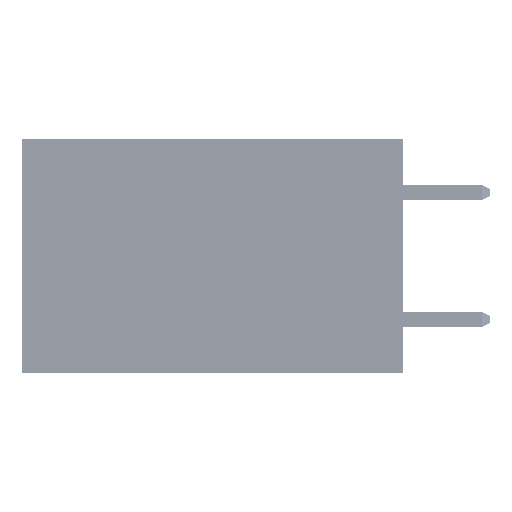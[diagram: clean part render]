
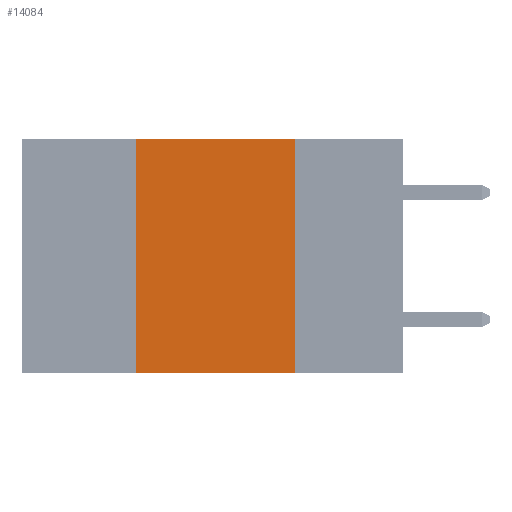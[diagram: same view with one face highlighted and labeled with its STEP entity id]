
A CAD part, left-side view. The second image highlights one B-rep face of the part: STEP entity #14084.
In plain terms, the highlighted planar face has unit normal (-1, 0, 0).
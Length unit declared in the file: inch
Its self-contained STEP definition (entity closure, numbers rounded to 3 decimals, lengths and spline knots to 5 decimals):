
#609 = CARTESIAN_POINT ( 'NONE',  ( 0., 0.17, 0. ) ) ;
#5768 = LINE ( 'NONE', #37172, #46860 ) ;
#5972 = ORIENTED_EDGE ( 'NONE', *, *, #36355, .F. ) ;
#6825 = ORIENTED_EDGE ( 'NONE', *, *, #26324, .F. ) ;
#8878 = CARTESIAN_POINT ( 'NONE',  ( 0., 0.17, 0. ) ) ;
#10198 = AXIS2_PLACEMENT_3D ( 'NONE', #22796, #34400, #19366 ) ;
#10320 = FACE_OUTER_BOUND ( 'NONE', #25816, .T. ) ;
#14084 = ADVANCED_FACE ( 'NONE', ( #10320 ), #42012, .F. ) ;
#14096 = VERTEX_POINT ( 'NONE', #609 ) ;
#15864 = CARTESIAN_POINT ( 'NONE',  ( 0., 0.42, 0. ) ) ;
#15959 = CARTESIAN_POINT ( 'NONE',  ( 0., 0.42, 0. ) ) ;
#18615 = VERTEX_POINT ( 'NONE', #35736 ) ;
#19366 = DIRECTION ( 'NONE',  ( 0., 0., -1. ) ) ;
#19368 = CARTESIAN_POINT ( 'NONE',  ( 0., 0.6, 0. ) ) ;
#19670 = VERTEX_POINT ( 'NONE', #29926 ) ;
#19706 = EDGE_CURVE ( 'NONE', #18615, #19670, #5768, .T. ) ;
#20727 = DIRECTION ( 'NONE',  ( 0., 0., -1. ) ) ;
#22165 = LINE ( 'NONE', #19368, #46283 ) ;
#22796 = CARTESIAN_POINT ( 'NONE',  ( 0., 0.6, 0. ) ) ;
#23823 = DIRECTION ( 'NONE',  ( 0., 0., 1. ) ) ;
#23917 = LINE ( 'NONE', #15864, #33580 ) ;
#25816 = EDGE_LOOP ( 'NONE', ( #42036, #5972, #6825, #30201 ) ) ;
#26324 = EDGE_CURVE ( 'NONE', #18615, #44539, #23917, .T. ) ;
#26517 = DIRECTION ( 'NONE',  ( 0., -1., 0. ) ) ;
#28520 = VECTOR ( 'NONE', #20727, 39.37008 ) ;
#28904 = EDGE_CURVE ( 'NONE', #14096, #19670, #37559, .T. ) ;
#29926 = CARTESIAN_POINT ( 'NONE',  ( 0., 0.17, -0.37 ) ) ;
#30201 = ORIENTED_EDGE ( 'NONE', *, *, #19706, .T. ) ;
#33580 = VECTOR ( 'NONE', #23823, 39.37008 ) ;
#33769 = DIRECTION ( 'NONE',  ( 0., -1., 0. ) ) ;
#34400 = DIRECTION ( 'NONE',  ( 1., 0., 0. ) ) ;
#35736 = CARTESIAN_POINT ( 'NONE',  ( 0., 0.42, -0.37 ) ) ;
#36355 = EDGE_CURVE ( 'NONE', #44539, #14096, #22165, .T. ) ;
#37172 = CARTESIAN_POINT ( 'NONE',  ( 0., 0.6, -0.37 ) ) ;
#37559 = LINE ( 'NONE', #8878, #28520 ) ;
#42012 = PLANE ( 'NONE',  #10198 ) ;
#42036 = ORIENTED_EDGE ( 'NONE', *, *, #28904, .F. ) ;
#44539 = VERTEX_POINT ( 'NONE', #15959 ) ;
#46283 = VECTOR ( 'NONE', #26517, 39.37008 ) ;
#46860 = VECTOR ( 'NONE', #33769, 39.37008 ) ;
